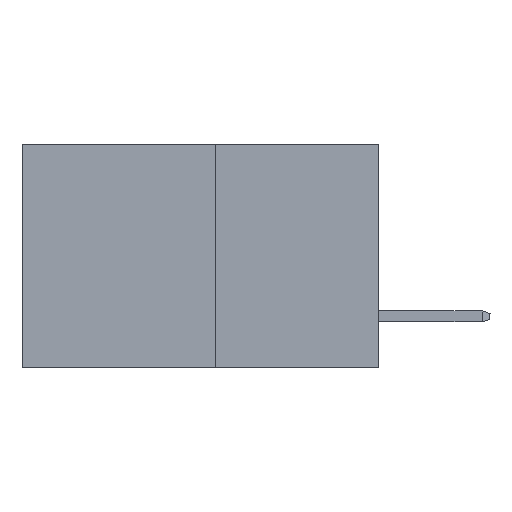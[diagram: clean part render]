
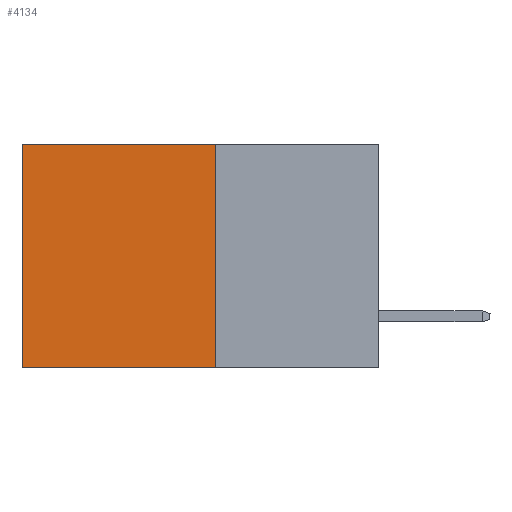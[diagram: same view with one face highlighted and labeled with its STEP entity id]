
A CAD part, left-side view. The second image highlights one B-rep face of the part: STEP entity #4134.
In plain terms, the highlighted planar face has unit normal (-1, 0, 0).
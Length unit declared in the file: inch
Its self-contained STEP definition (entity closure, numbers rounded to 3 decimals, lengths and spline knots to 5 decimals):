
#73 = EDGE_CURVE ( 'NONE', #13190, #11551, #1453, .T. ) ;
#779 = LINE ( 'NONE', #5930, #3598 ) ;
#1006 = EDGE_CURVE ( 'NONE', #11551, #1686, #1451, .T. ) ;
#1451 = LINE ( 'NONE', #7088, #9709 ) ;
#1453 = LINE ( 'NONE', #12917, #12209 ) ;
#1686 = VERTEX_POINT ( 'NONE', #12561 ) ;
#2656 = EDGE_CURVE ( 'NONE', #13190, #10076, #779, .T. ) ;
#2772 = CARTESIAN_POINT ( 'NONE',  ( 0.277, 0.27, 0. ) ) ;
#3598 = VECTOR ( 'NONE', #13257, 39.37008 ) ;
#4134 = ADVANCED_FACE ( 'NONE', ( #8525 ), #10299, .F. ) ;
#4600 = DIRECTION ( 'NONE',  ( 0., 0., -1. ) ) ;
#5365 = LINE ( 'NONE', #7788, #7801 ) ;
#5930 = CARTESIAN_POINT ( 'NONE',  ( 0.277, 0.27, -0.37 ) ) ;
#6497 = ORIENTED_EDGE ( 'NONE', *, *, #1006, .T. ) ;
#6661 = AXIS2_PLACEMENT_3D ( 'NONE', #10248, #10159, #10125 ) ;
#6819 = ORIENTED_EDGE ( 'NONE', *, *, #2656, .F. ) ;
#7088 = CARTESIAN_POINT ( 'NONE',  ( 0.277, 0.59, -0.37 ) ) ;
#7788 = CARTESIAN_POINT ( 'NONE',  ( 0.277, 0.27, -0.37 ) ) ;
#7801 = VECTOR ( 'NONE', #8796, 39.37008 ) ;
#8095 = EDGE_CURVE ( 'NONE', #10076, #1686, #5365, .T. ) ;
#8525 = FACE_OUTER_BOUND ( 'NONE', #11901, .T. ) ;
#8796 = DIRECTION ( 'NONE',  ( 0., 1., 0. ) ) ;
#8935 = CARTESIAN_POINT ( 'NONE',  ( 0.277, 0.59, 0. ) ) ;
#9249 = ORIENTED_EDGE ( 'NONE', *, *, #8095, .F. ) ;
#9564 = ORIENTED_EDGE ( 'NONE', *, *, #73, .T. ) ;
#9709 = VECTOR ( 'NONE', #4600, 39.37008 ) ;
#10076 = VERTEX_POINT ( 'NONE', #12765 ) ;
#10125 = DIRECTION ( 'NONE',  ( 0., 0., -1. ) ) ;
#10159 = DIRECTION ( 'NONE',  ( 1., 0., 0. ) ) ;
#10248 = CARTESIAN_POINT ( 'NONE',  ( 0.277, 0.27, -0.37 ) ) ;
#10299 = PLANE ( 'NONE',  #6661 ) ;
#11551 = VERTEX_POINT ( 'NONE', #8935 ) ;
#11901 = EDGE_LOOP ( 'NONE', ( #6497, #9249, #6819, #9564 ) ) ;
#12209 = VECTOR ( 'NONE', #12806, 39.37008 ) ;
#12561 = CARTESIAN_POINT ( 'NONE',  ( 0.277, 0.59, -0.37 ) ) ;
#12765 = CARTESIAN_POINT ( 'NONE',  ( 0.277, 0.27, -0.37 ) ) ;
#12806 = DIRECTION ( 'NONE',  ( 0., 1., 0. ) ) ;
#12917 = CARTESIAN_POINT ( 'NONE',  ( 0.277, 0.27, 0. ) ) ;
#13190 = VERTEX_POINT ( 'NONE', #2772 ) ;
#13257 = DIRECTION ( 'NONE',  ( 0., 0., -1. ) ) ;
